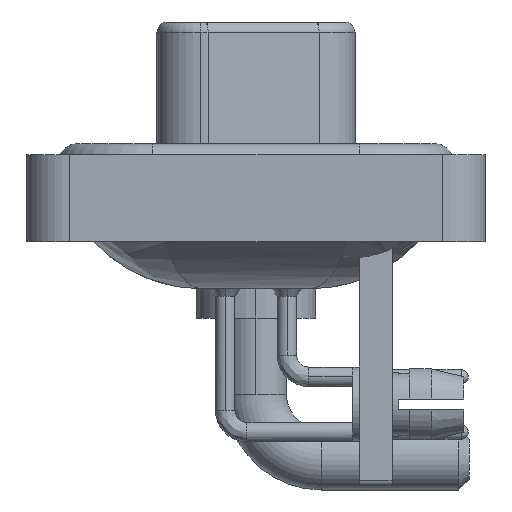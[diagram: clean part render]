
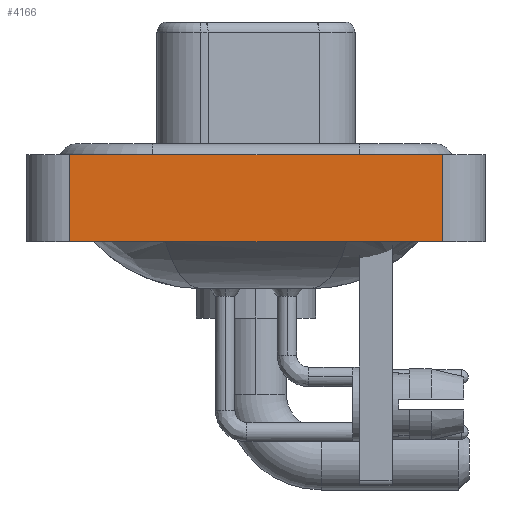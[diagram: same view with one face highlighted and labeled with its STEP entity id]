
A CAD part, left-side view. The second image highlights one B-rep face of the part: STEP entity #4166.
In plain terms, the highlighted planar face has unit normal (-1, 0, 0).
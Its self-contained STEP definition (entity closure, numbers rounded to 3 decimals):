
#217 = LINE ( 'NONE', #31740, #25734 ) ;
#553 = DIRECTION ( 'NONE',  ( -1., 0., 0. ) ) ;
#3501 = VERTEX_POINT ( 'NONE', #9354 ) ;
#3707 = ORIENTED_EDGE ( 'NONE', *, *, #20412, .F. ) ;
#4166 = ADVANCED_FACE ( 'NONE', ( #24801 ), #12802, .T. ) ;
#4219 = ORIENTED_EDGE ( 'NONE', *, *, #8857, .T. ) ;
#6856 = VECTOR ( 'NONE', #11243, 1000. ) ;
#6889 = VERTEX_POINT ( 'NONE', #30282 ) ;
#7947 = VECTOR ( 'NONE', #28294, 1000. ) ;
#8857 = EDGE_CURVE ( 'NONE', #6889, #25566, #27821, .T. ) ;
#9146 = CARTESIAN_POINT ( 'NONE',  ( -7.35, 8.55, -3.6 ) ) ;
#9354 = CARTESIAN_POINT ( 'NONE',  ( -7.35, 8.55, 0.4 ) ) ;
#10056 = DIRECTION ( 'NONE',  ( 0., -1., 0. ) ) ;
#11188 = EDGE_LOOP ( 'NONE', ( #4219, #3707, #11969, #16427 ) ) ;
#11243 = DIRECTION ( 'NONE',  ( 0., 0., 1. ) ) ;
#11614 = CARTESIAN_POINT ( 'NONE',  ( -7.35, -8.55, 0.4 ) ) ;
#11969 = ORIENTED_EDGE ( 'NONE', *, *, #29029, .F. ) ;
#12802 = PLANE ( 'NONE',  #27908 ) ;
#15688 = VECTOR ( 'NONE', #15761, 1000. ) ;
#15761 = DIRECTION ( 'NONE',  ( 0., -1., 0. ) ) ;
#16427 = ORIENTED_EDGE ( 'NONE', *, *, #25816, .T. ) ;
#20412 = EDGE_CURVE ( 'NONE', #3501, #25566, #217, .T. ) ;
#22694 = CARTESIAN_POINT ( 'NONE',  ( -7.35, -8.55, -3.6 ) ) ;
#24801 = FACE_OUTER_BOUND ( 'NONE', #11188, .T. ) ;
#25176 = CARTESIAN_POINT ( 'NONE',  ( -7.35, 8.55, -3.6 ) ) ;
#25566 = VERTEX_POINT ( 'NONE', #11614 ) ;
#25700 = CARTESIAN_POINT ( 'NONE',  ( -7.35, -8.55, -3.6 ) ) ;
#25734 = VECTOR ( 'NONE', #10056, 1000. ) ;
#25816 = EDGE_CURVE ( 'NONE', #28834, #6889, #30362, .T. ) ;
#26470 = LINE ( 'NONE', #9146, #6856 ) ;
#27821 = LINE ( 'NONE', #25700, #7947 ) ;
#27908 = AXIS2_PLACEMENT_3D ( 'NONE', #22694, #553, #30135 ) ;
#28294 = DIRECTION ( 'NONE',  ( 0., 0., 1. ) ) ;
#28834 = VERTEX_POINT ( 'NONE', #25176 ) ;
#29029 = EDGE_CURVE ( 'NONE', #28834, #3501, #26470, .T. ) ;
#30135 = DIRECTION ( 'NONE',  ( 0., 0., 1. ) ) ;
#30282 = CARTESIAN_POINT ( 'NONE',  ( -7.35, -8.55, -3.6 ) ) ;
#30362 = LINE ( 'NONE', #30996, #15688 ) ;
#30996 = CARTESIAN_POINT ( 'NONE',  ( -7.35, -8.55, -3.6 ) ) ;
#31740 = CARTESIAN_POINT ( 'NONE',  ( -7.35, -8.55, 0.4 ) ) ;
